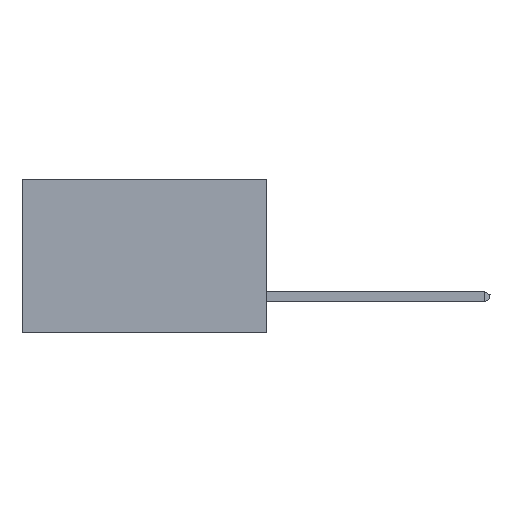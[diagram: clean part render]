
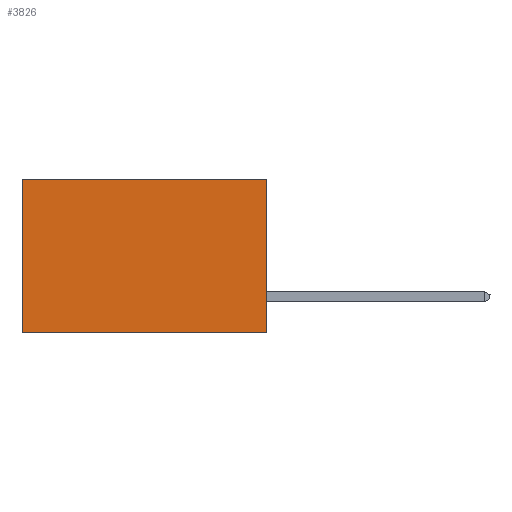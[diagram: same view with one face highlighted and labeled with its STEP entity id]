
A CAD part, left-side view. The second image highlights one B-rep face of the part: STEP entity #3826.
In plain terms, the highlighted planar face has unit normal (-1, 0, 0).
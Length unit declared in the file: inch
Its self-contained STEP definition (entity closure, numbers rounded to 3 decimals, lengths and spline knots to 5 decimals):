
#37 = DIRECTION ( 'NONE',  ( 0., 0., -1. ) ) ;
#157 = LINE ( 'NONE', #7072, #5600 ) ;
#329 = CARTESIAN_POINT ( 'NONE',  ( 0.2875, 0.6, -0.375 ) ) ;
#344 = VECTOR ( 'NONE', #9487, 39.37008 ) ;
#940 = ORIENTED_EDGE ( 'NONE', *, *, #11354, .T. ) ;
#1518 = LINE ( 'NONE', #5491, #344 ) ;
#1835 = DIRECTION ( 'NONE',  ( 1., 0., 0. ) ) ;
#1902 = PLANE ( 'NONE',  #2642 ) ;
#2041 = ORIENTED_EDGE ( 'NONE', *, *, #7767, .T. ) ;
#2642 = AXIS2_PLACEMENT_3D ( 'NONE', #12856, #1835, #7904 ) ;
#2991 = ORIENTED_EDGE ( 'NONE', *, *, #12183, .F. ) ;
#3184 = LINE ( 'NONE', #11148, #4794 ) ;
#3730 = EDGE_CURVE ( 'NONE', #6681, #7200, #1518, .T. ) ;
#3826 = ADVANCED_FACE ( 'NONE', ( #6728 ), #1902, .F. ) ;
#4794 = VECTOR ( 'NONE', #37, 39.37008 ) ;
#5119 = CARTESIAN_POINT ( 'NONE',  ( 0.2875, 0., -0.375 ) ) ;
#5491 = CARTESIAN_POINT ( 'NONE',  ( 0.2875, 0., -0.375 ) ) ;
#5600 = VECTOR ( 'NONE', #8201, 39.37008 ) ;
#6226 = VERTEX_POINT ( 'NONE', #9134 ) ;
#6326 = LINE ( 'NONE', #7185, #9180 ) ;
#6681 = VERTEX_POINT ( 'NONE', #5119 ) ;
#6728 = FACE_OUTER_BOUND ( 'NONE', #11424, .T. ) ;
#7072 = CARTESIAN_POINT ( 'NONE',  ( 0.2875, 0.6, -0.375 ) ) ;
#7076 = ORIENTED_EDGE ( 'NONE', *, *, #3730, .F. ) ;
#7185 = CARTESIAN_POINT ( 'NONE',  ( 0.2875, 0., 0. ) ) ;
#7200 = VERTEX_POINT ( 'NONE', #329 ) ;
#7767 = EDGE_CURVE ( 'NONE', #6226, #7200, #157, .T. ) ;
#7904 = DIRECTION ( 'NONE',  ( 0., 0., -1. ) ) ;
#8201 = DIRECTION ( 'NONE',  ( 0., 0., -1. ) ) ;
#8602 = VERTEX_POINT ( 'NONE', #10720 ) ;
#9097 = DIRECTION ( 'NONE',  ( 0., 1., 0. ) ) ;
#9134 = CARTESIAN_POINT ( 'NONE',  ( 0.2875, 0.6, 0. ) ) ;
#9180 = VECTOR ( 'NONE', #9097, 39.37008 ) ;
#9487 = DIRECTION ( 'NONE',  ( 0., 1., 0. ) ) ;
#10720 = CARTESIAN_POINT ( 'NONE',  ( 0.2875, 0., 0. ) ) ;
#11148 = CARTESIAN_POINT ( 'NONE',  ( 0.2875, 0., -0.375 ) ) ;
#11354 = EDGE_CURVE ( 'NONE', #8602, #6226, #6326, .T. ) ;
#11424 = EDGE_LOOP ( 'NONE', ( #2041, #7076, #2991, #940 ) ) ;
#12183 = EDGE_CURVE ( 'NONE', #8602, #6681, #3184, .T. ) ;
#12856 = CARTESIAN_POINT ( 'NONE',  ( 0.2875, 0., -0.375 ) ) ;
